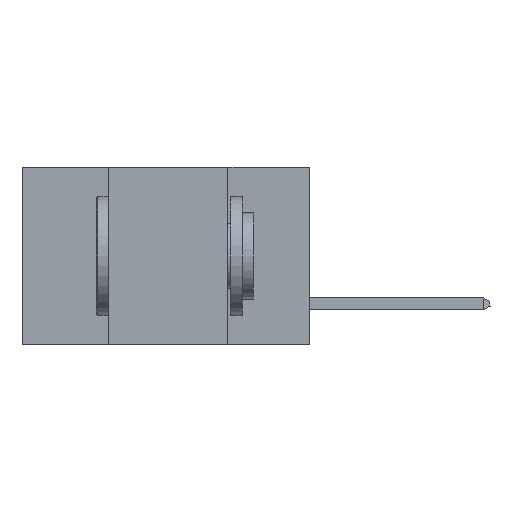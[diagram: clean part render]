
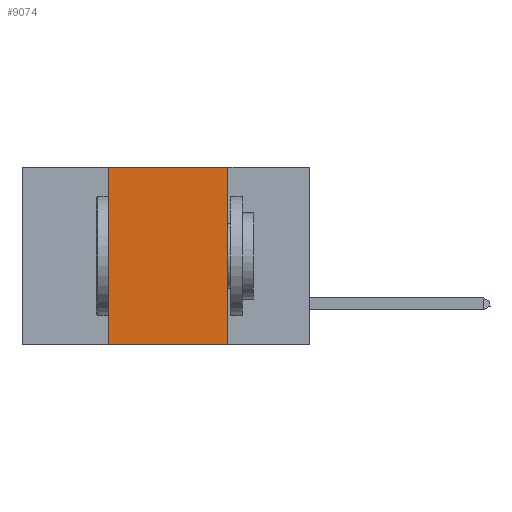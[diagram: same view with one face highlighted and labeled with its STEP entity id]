
A CAD part, left-side view. The second image highlights one B-rep face of the part: STEP entity #9074.
In plain terms, the highlighted planar face has unit normal (-1, 0, 0).
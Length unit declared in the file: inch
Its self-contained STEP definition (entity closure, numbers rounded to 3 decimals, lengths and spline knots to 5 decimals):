
#1423 = VERTEX_POINT ( 'NONE', #9355 ) ;
#1488 = CARTESIAN_POINT ( 'NONE',  ( 0., 0.42, 0. ) ) ;
#2878 = LINE ( 'NONE', #14625, #7121 ) ;
#3134 = CARTESIAN_POINT ( 'NONE',  ( 0., 0.42, -0.37 ) ) ;
#4628 = VERTEX_POINT ( 'NONE', #10666 ) ;
#5338 = VECTOR ( 'NONE', #8130, 39.37008 ) ;
#5798 = CARTESIAN_POINT ( 'NONE',  ( 0., 0.42, 0. ) ) ;
#5902 = VECTOR ( 'NONE', #10324, 39.37008 ) ;
#7121 = VECTOR ( 'NONE', #17413, 39.37008 ) ;
#7215 = VERTEX_POINT ( 'NONE', #3134 ) ;
#7455 = DIRECTION ( 'NONE',  ( 1., 0., 0. ) ) ;
#8130 = DIRECTION ( 'NONE',  ( 0., -1., 0. ) ) ;
#8248 = EDGE_LOOP ( 'NONE', ( #19808, #8892, #13604, #15575 ) ) ;
#8305 = LINE ( 'NONE', #12352, #5902 ) ;
#8892 = ORIENTED_EDGE ( 'NONE', *, *, #23579, .F. ) ;
#9074 = ADVANCED_FACE ( 'NONE', ( #14536 ), #9257, .F. ) ;
#9257 = PLANE ( 'NONE',  #24855 ) ;
#9345 = DIRECTION ( 'NONE',  ( 0., 0., -1. ) ) ;
#9355 = CARTESIAN_POINT ( 'NONE',  ( 0., 0.17, 0. ) ) ;
#9622 = LINE ( 'NONE', #5798, #11147 ) ;
#10324 = DIRECTION ( 'NONE',  ( 0., 0., -1. ) ) ;
#10666 = CARTESIAN_POINT ( 'NONE',  ( 0., 0.17, -0.37 ) ) ;
#11147 = VECTOR ( 'NONE', #13572, 39.37008 ) ;
#11272 = VERTEX_POINT ( 'NONE', #1488 ) ;
#12352 = CARTESIAN_POINT ( 'NONE',  ( 0., 0.17, 0. ) ) ;
#12542 = EDGE_CURVE ( 'NONE', #7215, #4628, #18917, .T. ) ;
#13572 = DIRECTION ( 'NONE',  ( 0., 0., 1. ) ) ;
#13604 = ORIENTED_EDGE ( 'NONE', *, *, #20708, .F. ) ;
#14536 = FACE_OUTER_BOUND ( 'NONE', #8248, .T. ) ;
#14625 = CARTESIAN_POINT ( 'NONE',  ( 0., 0.6, 0. ) ) ;
#15575 = ORIENTED_EDGE ( 'NONE', *, *, #12542, .T. ) ;
#16952 = EDGE_CURVE ( 'NONE', #1423, #4628, #8305, .T. ) ;
#17413 = DIRECTION ( 'NONE',  ( 0., -1., 0. ) ) ;
#17847 = CARTESIAN_POINT ( 'NONE',  ( 0., 0.6, -0.37 ) ) ;
#18917 = LINE ( 'NONE', #17847, #5338 ) ;
#19808 = ORIENTED_EDGE ( 'NONE', *, *, #16952, .F. ) ;
#20708 = EDGE_CURVE ( 'NONE', #7215, #11272, #9622, .T. ) ;
#22782 = CARTESIAN_POINT ( 'NONE',  ( 0., 0.6, 0. ) ) ;
#23579 = EDGE_CURVE ( 'NONE', #11272, #1423, #2878, .T. ) ;
#24855 = AXIS2_PLACEMENT_3D ( 'NONE', #22782, #7455, #9345 ) ;
